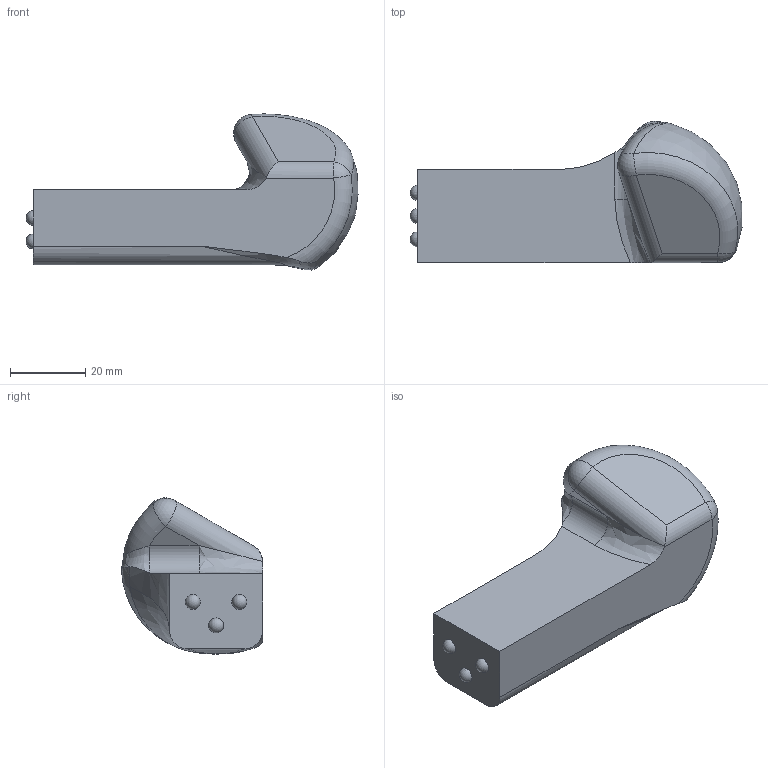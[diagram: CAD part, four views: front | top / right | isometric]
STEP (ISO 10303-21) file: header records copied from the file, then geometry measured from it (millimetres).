
FILE_DESCRIPTION (( 'STEP AP214' ), '1' );
FILE_NAME ('Bipod_Right_Part_1_V2.step', '2016-01-25T18:17:16', ( 'WarFairy' ), ( '' ), 'SwSTEP 2.0', 'SolidWorks 2015', '' );
FILE_SCHEMA (( 'AUTOMOTIVE_DESIGN' ));
Length unit declared in the file: inch
Products named in the file (1): Bipod_Right_Part_1_V2
Bounding box: 88.44 x 37.62 x 41.6 mm (x, y, z)
Volume: 55610.1 mm3; surface area: 9742.4 mm2
Topology: 1 solids, 1 shells, 32 faces, 82 edges, 48 vertices
Faces by surface type: bspline 11, plane 7, sphere 6, cylinder 5, torus 3
Entity records: 1685 total; most frequent: CARTESIAN_POINT 1030, ORIENTED_EDGE 138, DIRECTION 110, EDGE_CURVE 69, AXIS2_PLACEMENT_3D 47, VERTEX_POINT 42, EDGE_LOOP 35, ADVANCED_FACE 32
